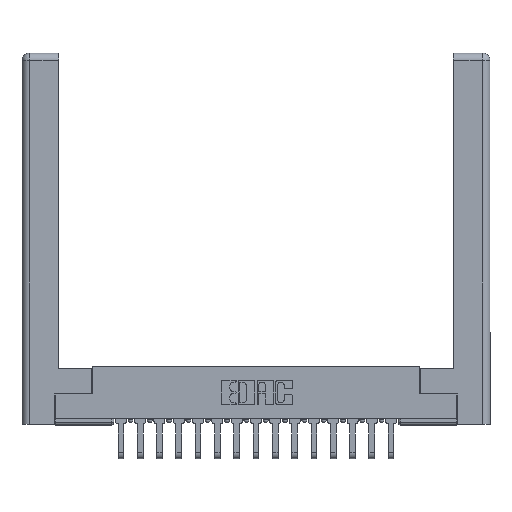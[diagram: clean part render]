
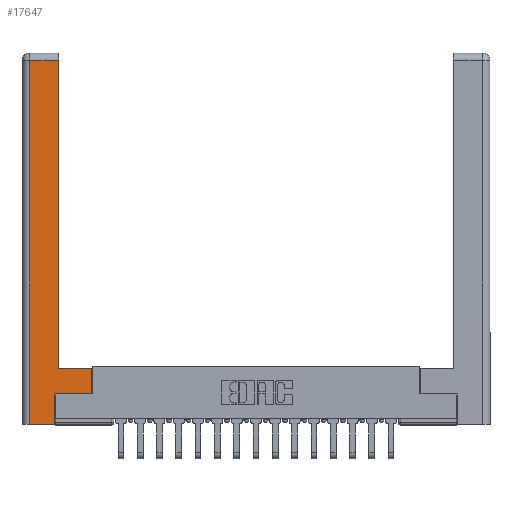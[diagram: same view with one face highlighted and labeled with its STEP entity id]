
A CAD part, top view. The second image highlights one B-rep face of the part: STEP entity #17647.
In plain terms, the highlighted planar face has unit normal (0, 0, 1).
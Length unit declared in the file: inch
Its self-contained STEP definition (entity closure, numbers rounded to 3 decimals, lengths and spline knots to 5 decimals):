
#284 = CARTESIAN_POINT ( 'NONE',  ( 0.295, 0.45, 0. ) ) ;
#411 = CARTESIAN_POINT ( 'NONE',  ( 0.265, 0., 0. ) ) ;
#768 = VERTEX_POINT ( 'NONE', #8441 ) ;
#925 = LINE ( 'NONE', #3930, #6884 ) ;
#1569 = LINE ( 'NONE', #4127, #9793 ) ;
#2020 = ORIENTED_EDGE ( 'NONE', *, *, #12876, .T. ) ;
#2138 = LINE ( 'NONE', #8234, #7880 ) ;
#3100 = EDGE_CURVE ( 'NONE', #4177, #9810, #8327, .T. ) ;
#3246 = CARTESIAN_POINT ( 'NONE',  ( 0.565, 0.45, 0. ) ) ;
#3264 = VERTEX_POINT ( 'NONE', #9862 ) ;
#3431 = EDGE_CURVE ( 'NONE', #3264, #10913, #10583, .T. ) ;
#3930 = CARTESIAN_POINT ( 'NONE',  ( 0.0615, 0., 0. ) ) ;
#4064 = DIRECTION ( 'NONE',  ( -1., 0., 0. ) ) ;
#4127 = CARTESIAN_POINT ( 'NONE',  ( 0.0615, 2.94, 0. ) ) ;
#4177 = VERTEX_POINT ( 'NONE', #8552 ) ;
#4372 = DIRECTION ( 'NONE',  ( -1., 0., 0. ) ) ;
#4440 = VECTOR ( 'NONE', #4372, 39.37008 ) ;
#4459 = ORIENTED_EDGE ( 'NONE', *, *, #3431, .T. ) ;
#4537 = CARTESIAN_POINT ( 'NONE',  ( 0.265, 0.245, 0. ) ) ;
#4552 = CARTESIAN_POINT ( 'NONE',  ( 0.295, 0.45, 0. ) ) ;
#4833 = DIRECTION ( 'NONE',  ( 0., 0., -1. ) ) ;
#5144 = DIRECTION ( 'NONE',  ( 0., 1., 0. ) ) ;
#5475 = DIRECTION ( 'NONE',  ( 1., 0., 0. ) ) ;
#6043 = PLANE ( 'NONE',  #10285 ) ;
#6323 = CARTESIAN_POINT ( 'NONE',  ( 0.295, 2.94, 0. ) ) ;
#6884 = VECTOR ( 'NONE', #14265, 39.37008 ) ;
#7027 = CARTESIAN_POINT ( 'NONE',  ( 0.295, 3., 0. ) ) ;
#7212 = VERTEX_POINT ( 'NONE', #15124 ) ;
#7621 = ORIENTED_EDGE ( 'NONE', *, *, #13797, .T. ) ;
#7810 = LINE ( 'NONE', #8320, #9175 ) ;
#7880 = VECTOR ( 'NONE', #5475, 39.37008 ) ;
#8234 = CARTESIAN_POINT ( 'NONE',  ( 0.565, 0.245, 0. ) ) ;
#8320 = CARTESIAN_POINT ( 'NONE',  ( 0.265, 0.245, 0. ) ) ;
#8327 = LINE ( 'NONE', #4552, #4440 ) ;
#8345 = VERTEX_POINT ( 'NONE', #6323 ) ;
#8441 = CARTESIAN_POINT ( 'NONE',  ( 0.0615, 2.94, 0. ) ) ;
#8552 = CARTESIAN_POINT ( 'NONE',  ( 0.565, 0.45, 0. ) ) ;
#8632 = EDGE_LOOP ( 'NONE', ( #18093, #16531, #7621, #4459, #9993, #15522, #2020, #13211 ) ) ;
#8831 = EDGE_CURVE ( 'NONE', #10913, #10873, #7810, .T. ) ;
#9003 = CARTESIAN_POINT ( 'NONE',  ( 0.265, 0., 0. ) ) ;
#9175 = VECTOR ( 'NONE', #18657, 39.37008 ) ;
#9793 = VECTOR ( 'NONE', #4064, 39.37008 ) ;
#9810 = VERTEX_POINT ( 'NONE', #284 ) ;
#9862 = CARTESIAN_POINT ( 'NONE',  ( 0.0615, 0., 0. ) ) ;
#9993 = ORIENTED_EDGE ( 'NONE', *, *, #8831, .T. ) ;
#10246 = EDGE_CURVE ( 'NONE', #8345, #768, #1569, .T. ) ;
#10285 = AXIS2_PLACEMENT_3D ( 'NONE', #16260, #4833, #13582 ) ;
#10323 = FACE_OUTER_BOUND ( 'NONE', #8632, .T. ) ;
#10576 = LINE ( 'NONE', #3246, #16744 ) ;
#10583 = LINE ( 'NONE', #411, #12181 ) ;
#10873 = VERTEX_POINT ( 'NONE', #4537 ) ;
#10913 = VERTEX_POINT ( 'NONE', #9003 ) ;
#10954 = VECTOR ( 'NONE', #17162, 39.37008 ) ;
#11222 = EDGE_CURVE ( 'NONE', #10873, #7212, #2138, .T. ) ;
#12181 = VECTOR ( 'NONE', #13694, 39.37008 ) ;
#12876 = EDGE_CURVE ( 'NONE', #7212, #4177, #10576, .T. ) ;
#13211 = ORIENTED_EDGE ( 'NONE', *, *, #3100, .T. ) ;
#13582 = DIRECTION ( 'NONE',  ( -1., 0., 0. ) ) ;
#13694 = DIRECTION ( 'NONE',  ( 1., 0., 0. ) ) ;
#13797 = EDGE_CURVE ( 'NONE', #768, #3264, #925, .T. ) ;
#14265 = DIRECTION ( 'NONE',  ( 0., -1., 0. ) ) ;
#14637 = EDGE_CURVE ( 'NONE', #9810, #8345, #14839, .T. ) ;
#14839 = LINE ( 'NONE', #7027, #10954 ) ;
#15124 = CARTESIAN_POINT ( 'NONE',  ( 0.565, 0.245, 0. ) ) ;
#15522 = ORIENTED_EDGE ( 'NONE', *, *, #11222, .T. ) ;
#16260 = CARTESIAN_POINT ( 'NONE',  ( 0., 0., 0. ) ) ;
#16531 = ORIENTED_EDGE ( 'NONE', *, *, #10246, .T. ) ;
#16744 = VECTOR ( 'NONE', #5144, 39.37008 ) ;
#17162 = DIRECTION ( 'NONE',  ( 0., 1., 0. ) ) ;
#17647 = ADVANCED_FACE ( 'NONE', ( #10323 ), #6043, .F. ) ;
#18093 = ORIENTED_EDGE ( 'NONE', *, *, #14637, .T. ) ;
#18657 = DIRECTION ( 'NONE',  ( 0., 1., 0. ) ) ;
